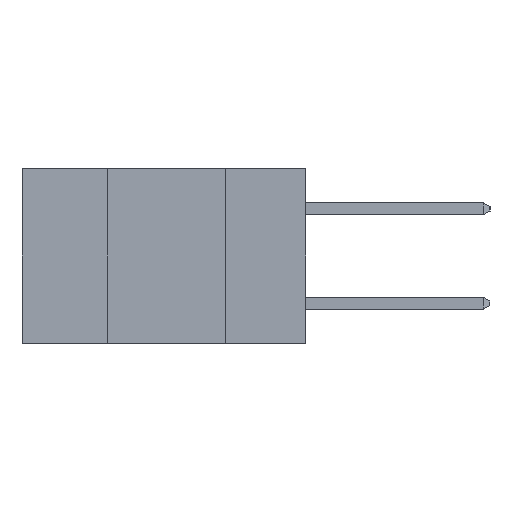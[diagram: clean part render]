
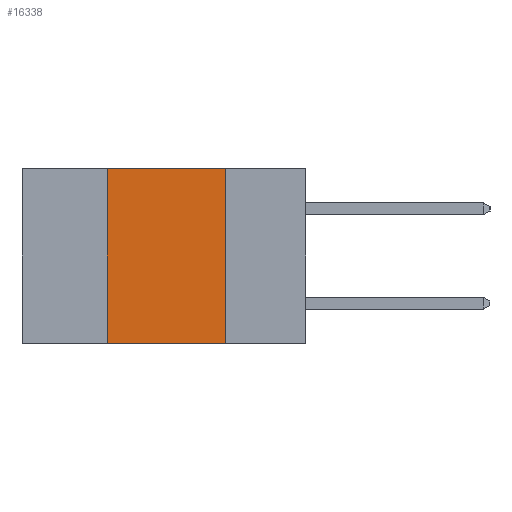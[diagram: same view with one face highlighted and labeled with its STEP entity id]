
A CAD part, left-side view. The second image highlights one B-rep face of the part: STEP entity #16338.
In plain terms, the highlighted planar face has unit normal (-1, 0, 0).
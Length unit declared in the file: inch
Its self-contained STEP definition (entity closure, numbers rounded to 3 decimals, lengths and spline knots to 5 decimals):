
#1423 = CARTESIAN_POINT ( 'NONE',  ( 0., 0.6, -0.37 ) ) ;
#1653 = LINE ( 'NONE', #18737, #12183 ) ;
#1675 = DIRECTION ( 'NONE',  ( 0., 0., 1. ) ) ;
#1723 = PLANE ( 'NONE',  #5819 ) ;
#3278 = EDGE_CURVE ( 'NONE', #15142, #13115, #16743, .T. ) ;
#4658 = ORIENTED_EDGE ( 'NONE', *, *, #3278, .F. ) ;
#5714 = VECTOR ( 'NONE', #1675, 39.37008 ) ;
#5819 = AXIS2_PLACEMENT_3D ( 'NONE', #10129, #17148, #12609 ) ;
#6090 = VECTOR ( 'NONE', #24298, 39.37008 ) ;
#6274 = DIRECTION ( 'NONE',  ( 0., -1., 0. ) ) ;
#7779 = FACE_OUTER_BOUND ( 'NONE', #14694, .T. ) ;
#8412 = ORIENTED_EDGE ( 'NONE', *, *, #13874, .F. ) ;
#9151 = CARTESIAN_POINT ( 'NONE',  ( 0., 0.42, -0.37 ) ) ;
#10129 = CARTESIAN_POINT ( 'NONE',  ( 0., 0.6, 0. ) ) ;
#11054 = EDGE_CURVE ( 'NONE', #22246, #16508, #15899, .T. ) ;
#11234 = VECTOR ( 'NONE', #6274, 39.37008 ) ;
#11355 = CARTESIAN_POINT ( 'NONE',  ( 0., 0.17, -0.37 ) ) ;
#12183 = VECTOR ( 'NONE', #18607, 39.37008 ) ;
#12609 = DIRECTION ( 'NONE',  ( 0., 0., -1. ) ) ;
#12932 = CARTESIAN_POINT ( 'NONE',  ( 0., 0.17, 0. ) ) ;
#13115 = VERTEX_POINT ( 'NONE', #12932 ) ;
#13444 = CARTESIAN_POINT ( 'NONE',  ( 0., 0.42, 0. ) ) ;
#13874 = EDGE_CURVE ( 'NONE', #22246, #15142, #26884, .T. ) ;
#14694 = EDGE_LOOP ( 'NONE', ( #18032, #4658, #8412, #17343 ) ) ;
#15142 = VERTEX_POINT ( 'NONE', #13444 ) ;
#15899 = LINE ( 'NONE', #1423, #6090 ) ;
#16338 = ADVANCED_FACE ( 'NONE', ( #7779 ), #1723, .F. ) ;
#16508 = VERTEX_POINT ( 'NONE', #11355 ) ;
#16743 = LINE ( 'NONE', #20592, #11234 ) ;
#17148 = DIRECTION ( 'NONE',  ( 1., 0., 0. ) ) ;
#17343 = ORIENTED_EDGE ( 'NONE', *, *, #11054, .T. ) ;
#18032 = ORIENTED_EDGE ( 'NONE', *, *, #26646, .F. ) ;
#18607 = DIRECTION ( 'NONE',  ( 0., 0., -1. ) ) ;
#18737 = CARTESIAN_POINT ( 'NONE',  ( 0., 0.17, -0.37 ) ) ;
#20592 = CARTESIAN_POINT ( 'NONE',  ( 0., 0.6, 0. ) ) ;
#22246 = VERTEX_POINT ( 'NONE', #9151 ) ;
#24298 = DIRECTION ( 'NONE',  ( 0., -1., 0. ) ) ;
#24542 = CARTESIAN_POINT ( 'NONE',  ( 0., 0.42, -0.37 ) ) ;
#26646 = EDGE_CURVE ( 'NONE', #13115, #16508, #1653, .T. ) ;
#26884 = LINE ( 'NONE', #24542, #5714 ) ;
